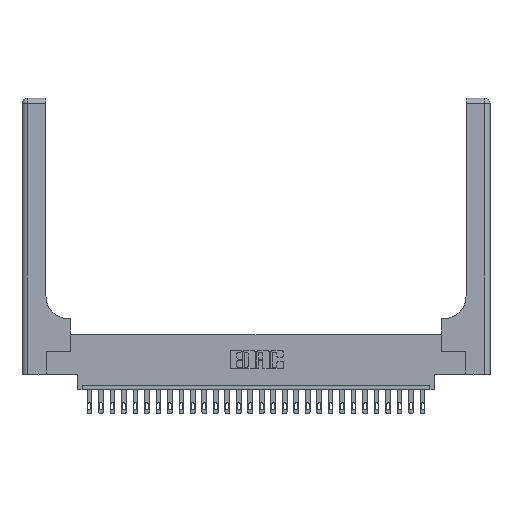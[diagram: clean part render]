
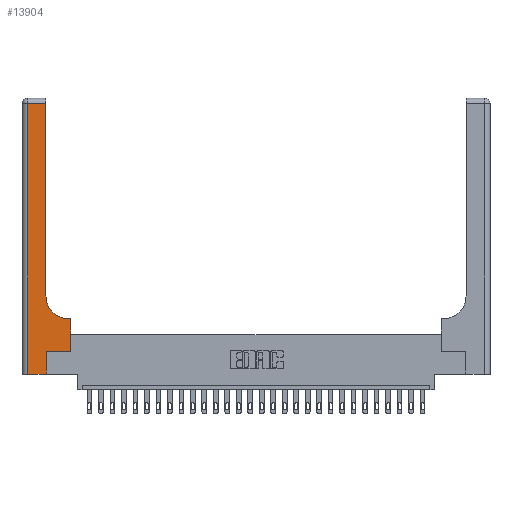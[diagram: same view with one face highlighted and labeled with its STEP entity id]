
A CAD part, top view. The second image highlights one B-rep face of the part: STEP entity #13904.
In plain terms, the highlighted planar face has unit normal (0, 0, 1).
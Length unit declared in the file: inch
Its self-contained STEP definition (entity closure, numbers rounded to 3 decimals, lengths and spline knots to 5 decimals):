
#771 = CARTESIAN_POINT ( 'NONE',  ( 0.528, 0.25, 0.37 ) ) ;
#1055 = CARTESIAN_POINT ( 'NONE',  ( 0.06, 0., 0.37 ) ) ;
#1218 = CARTESIAN_POINT ( 'NONE',  ( 0., 2.94, 0.37 ) ) ;
#1410 = VERTEX_POINT ( 'NONE', #9844 ) ;
#2022 = CARTESIAN_POINT ( 'NONE',  ( 0.06, 2.94, 0.37 ) ) ;
#3076 = CIRCLE ( 'NONE', #3491, 0.25 ) ;
#3094 = PLANE ( 'NONE',  #18135 ) ;
#3230 = CARTESIAN_POINT ( 'NONE',  ( 0., 3., 0.37 ) ) ;
#3435 = VERTEX_POINT ( 'NONE', #24562 ) ;
#3491 = AXIS2_PLACEMENT_3D ( 'NONE', #9125, #7026, #11219 ) ;
#3579 = DIRECTION ( 'NONE',  ( 1., 0., 0. ) ) ;
#3980 = VECTOR ( 'NONE', #9570, 39.37008 ) ;
#4049 = DIRECTION ( 'NONE',  ( 1., 0., 0. ) ) ;
#4113 = CARTESIAN_POINT ( 'NONE',  ( 0.26, 3., 0.37 ) ) ;
#4908 = EDGE_CURVE ( 'NONE', #23566, #1410, #24001, .T. ) ;
#5269 = LINE ( 'NONE', #13264, #3980 ) ;
#5685 = DIRECTION ( 'NONE',  ( -1., 0., 0. ) ) ;
#5756 = ORIENTED_EDGE ( 'NONE', *, *, #4908, .T. ) ;
#6068 = CARTESIAN_POINT ( 'NONE',  ( 0.26, 0.6, 0.37 ) ) ;
#6908 = EDGE_CURVE ( 'NONE', #11961, #8408, #20207, .T. ) ;
#7026 = DIRECTION ( 'NONE',  ( 0., 0., -1. ) ) ;
#7061 = EDGE_CURVE ( 'NONE', #3435, #16742, #14976, .T. ) ;
#7446 = LINE ( 'NONE', #15713, #19356 ) ;
#8379 = CARTESIAN_POINT ( 'NONE',  ( 0.265, 0., 0.37 ) ) ;
#8408 = VERTEX_POINT ( 'NONE', #22657 ) ;
#8849 = DIRECTION ( 'NONE',  ( -1., 0., 0. ) ) ;
#9125 = CARTESIAN_POINT ( 'NONE',  ( 0.51, 0.85, 0.37 ) ) ;
#9570 = DIRECTION ( 'NONE',  ( 0., 1., 0. ) ) ;
#9814 = CARTESIAN_POINT ( 'NONE',  ( 0., 0., 0.37 ) ) ;
#9844 = CARTESIAN_POINT ( 'NONE',  ( 0.51, 0.6, 0.37 ) ) ;
#9967 = DIRECTION ( 'NONE',  ( 0., 1., 0. ) ) ;
#10097 = ORIENTED_EDGE ( 'NONE', *, *, #11893, .T. ) ;
#10882 = ORIENTED_EDGE ( 'NONE', *, *, #13871, .T. ) ;
#11219 = DIRECTION ( 'NONE',  ( 1., 0., 0. ) ) ;
#11435 = LINE ( 'NONE', #1218, #20544 ) ;
#11453 = CARTESIAN_POINT ( 'NONE',  ( 0.265, 0., 0.37 ) ) ;
#11711 = DIRECTION ( 'NONE',  ( 0., 1., 0. ) ) ;
#11893 = EDGE_CURVE ( 'NONE', #23401, #23185, #21979, .T. ) ;
#11961 = VERTEX_POINT ( 'NONE', #13625 ) ;
#12467 = LINE ( 'NONE', #8379, #14039 ) ;
#12472 = ORIENTED_EDGE ( 'NONE', *, *, #7061, .T. ) ;
#13264 = CARTESIAN_POINT ( 'NONE',  ( 0.528, 0.25, 0.37 ) ) ;
#13314 = DIRECTION ( 'NONE',  ( 0., 0., -1. ) ) ;
#13625 = CARTESIAN_POINT ( 'NONE',  ( 0.26, 0.85, 0.37 ) ) ;
#13871 = EDGE_CURVE ( 'NONE', #1410, #11961, #3076, .T. ) ;
#13904 = ADVANCED_FACE ( 'NONE', ( #20897 ), #3094, .F. ) ;
#14039 = VECTOR ( 'NONE', #9967, 39.37008 ) ;
#14976 = LINE ( 'NONE', #15365, #21533 ) ;
#15365 = CARTESIAN_POINT ( 'NONE',  ( 0.265, 0.25, 0.37 ) ) ;
#15440 = DIRECTION ( 'NONE',  ( 0., -1., 0. ) ) ;
#15589 = VECTOR ( 'NONE', #5685, 39.37008 ) ;
#15713 = CARTESIAN_POINT ( 'NONE',  ( 0.06, 3., 0.37 ) ) ;
#16054 = EDGE_CURVE ( 'NONE', #8408, #21040, #11435, .T. ) ;
#16742 = VERTEX_POINT ( 'NONE', #771 ) ;
#18135 = AXIS2_PLACEMENT_3D ( 'NONE', #3230, #13314, #8849 ) ;
#18180 = VECTOR ( 'NONE', #11711, 39.37008 ) ;
#18817 = ORIENTED_EDGE ( 'NONE', *, *, #6908, .T. ) ;
#19356 = VECTOR ( 'NONE', #15440, 39.37008 ) ;
#19499 = ORIENTED_EDGE ( 'NONE', *, *, #21765, .T. ) ;
#20109 = ORIENTED_EDGE ( 'NONE', *, *, #24886, .T. ) ;
#20207 = LINE ( 'NONE', #4113, #18180 ) ;
#20544 = VECTOR ( 'NONE', #21370, 39.37008 ) ;
#20897 = FACE_OUTER_BOUND ( 'NONE', #22943, .T. ) ;
#21040 = VERTEX_POINT ( 'NONE', #2022 ) ;
#21370 = DIRECTION ( 'NONE',  ( -1., 0., 0. ) ) ;
#21533 = VECTOR ( 'NONE', #3579, 39.37008 ) ;
#21765 = EDGE_CURVE ( 'NONE', #16742, #23566, #5269, .T. ) ;
#21977 = CARTESIAN_POINT ( 'NONE',  ( 0.528, 0.6, 0.37 ) ) ;
#21979 = LINE ( 'NONE', #9814, #25243 ) ;
#22323 = EDGE_CURVE ( 'NONE', #21040, #23401, #7446, .T. ) ;
#22657 = CARTESIAN_POINT ( 'NONE',  ( 0.26, 2.94, 0.37 ) ) ;
#22943 = EDGE_LOOP ( 'NONE', ( #18817, #23561, #24238, #10097, #20109, #12472, #19499, #5756, #10882 ) ) ;
#23185 = VERTEX_POINT ( 'NONE', #11453 ) ;
#23401 = VERTEX_POINT ( 'NONE', #1055 ) ;
#23561 = ORIENTED_EDGE ( 'NONE', *, *, #16054, .T. ) ;
#23566 = VERTEX_POINT ( 'NONE', #21977 ) ;
#24001 = LINE ( 'NONE', #6068, #15589 ) ;
#24238 = ORIENTED_EDGE ( 'NONE', *, *, #22323, .T. ) ;
#24562 = CARTESIAN_POINT ( 'NONE',  ( 0.265, 0.25, 0.37 ) ) ;
#24886 = EDGE_CURVE ( 'NONE', #23185, #3435, #12467, .T. ) ;
#25243 = VECTOR ( 'NONE', #4049, 39.37008 ) ;
